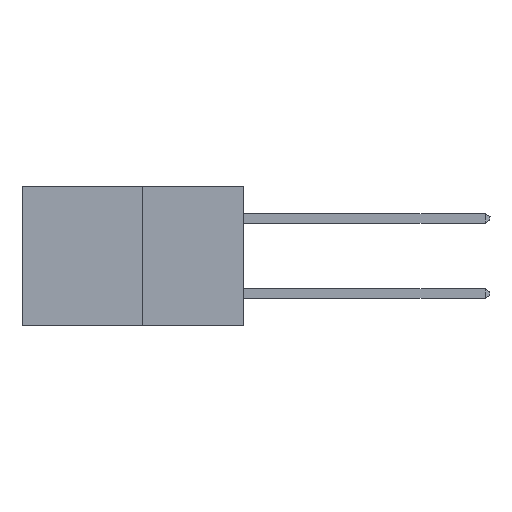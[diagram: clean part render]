
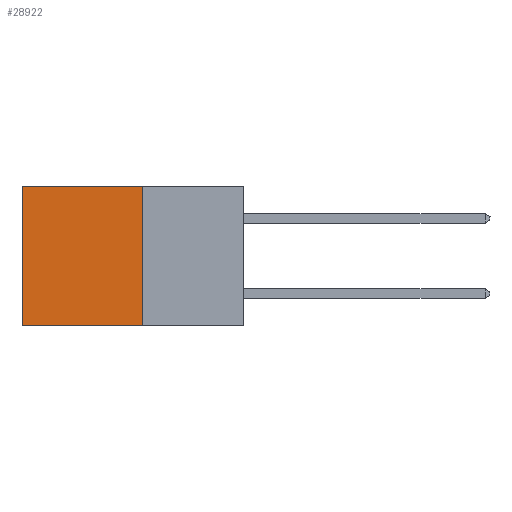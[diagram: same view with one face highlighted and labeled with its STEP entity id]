
A CAD part, left-side view. The second image highlights one B-rep face of the part: STEP entity #28922.
In plain terms, the highlighted planar face has unit normal (-1, 0, 0).
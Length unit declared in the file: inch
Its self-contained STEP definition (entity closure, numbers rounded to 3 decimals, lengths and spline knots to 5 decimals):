
#3131 = AXIS2_PLACEMENT_3D ( 'NONE', #15599, #7849, #26029 ) ;
#4768 = VECTOR ( 'NONE', #27327, 39.37008 ) ;
#5246 = LINE ( 'NONE', #26221, #18449 ) ;
#6425 = LINE ( 'NONE', #22226, #4768 ) ;
#7557 = VERTEX_POINT ( 'NONE', #31837 ) ;
#7715 = ORIENTED_EDGE ( 'NONE', *, *, #15139, .T. ) ;
#7849 = DIRECTION ( 'NONE',  ( 1., 0., 0. ) ) ;
#8227 = ORIENTED_EDGE ( 'NONE', *, *, #23034, .T. ) ;
#8614 = LINE ( 'NONE', #15072, #27663 ) ;
#9855 = DIRECTION ( 'NONE',  ( 0., 1., 0. ) ) ;
#10586 = VERTEX_POINT ( 'NONE', #14207 ) ;
#12923 = EDGE_LOOP ( 'NONE', ( #7715, #20934, #19734, #8227 ) ) ;
#14207 = CARTESIAN_POINT ( 'NONE',  ( 0.277, 0.27, 0. ) ) ;
#15072 = CARTESIAN_POINT ( 'NONE',  ( 0.277, 0.27, -0.37 ) ) ;
#15139 = EDGE_CURVE ( 'NONE', #19850, #7557, #5246, .T. ) ;
#15599 = CARTESIAN_POINT ( 'NONE',  ( 0.277, 0.27, -0.37 ) ) ;
#16473 = FACE_OUTER_BOUND ( 'NONE', #12923, .T. ) ;
#18449 = VECTOR ( 'NONE', #28783, 39.37008 ) ;
#19734 = ORIENTED_EDGE ( 'NONE', *, *, #24865, .F. ) ;
#19850 = VERTEX_POINT ( 'NONE', #24200 ) ;
#20934 = ORIENTED_EDGE ( 'NONE', *, *, #26971, .F. ) ;
#21469 = VECTOR ( 'NONE', #26788, 39.37008 ) ;
#22226 = CARTESIAN_POINT ( 'NONE',  ( 0.277, 0.27, 0. ) ) ;
#23034 = EDGE_CURVE ( 'NONE', #10586, #19850, #6425, .T. ) ;
#23492 = PLANE ( 'NONE',  #3131 ) ;
#24200 = CARTESIAN_POINT ( 'NONE',  ( 0.277, 0.59, 0. ) ) ;
#24213 = CARTESIAN_POINT ( 'NONE',  ( 0.277, 0.27, -0.37 ) ) ;
#24865 = EDGE_CURVE ( 'NONE', #10586, #29283, #29009, .T. ) ;
#26029 = DIRECTION ( 'NONE',  ( 0., 0., -1. ) ) ;
#26221 = CARTESIAN_POINT ( 'NONE',  ( 0.277, 0.59, -0.37 ) ) ;
#26788 = DIRECTION ( 'NONE',  ( 0., 0., -1. ) ) ;
#26971 = EDGE_CURVE ( 'NONE', #29283, #7557, #8614, .T. ) ;
#27327 = DIRECTION ( 'NONE',  ( 0., 1., 0. ) ) ;
#27348 = CARTESIAN_POINT ( 'NONE',  ( 0.277, 0.27, -0.37 ) ) ;
#27663 = VECTOR ( 'NONE', #9855, 39.37008 ) ;
#28783 = DIRECTION ( 'NONE',  ( 0., 0., -1. ) ) ;
#28922 = ADVANCED_FACE ( 'NONE', ( #16473 ), #23492, .F. ) ;
#29009 = LINE ( 'NONE', #24213, #21469 ) ;
#29283 = VERTEX_POINT ( 'NONE', #27348 ) ;
#31837 = CARTESIAN_POINT ( 'NONE',  ( 0.277, 0.59, -0.37 ) ) ;
